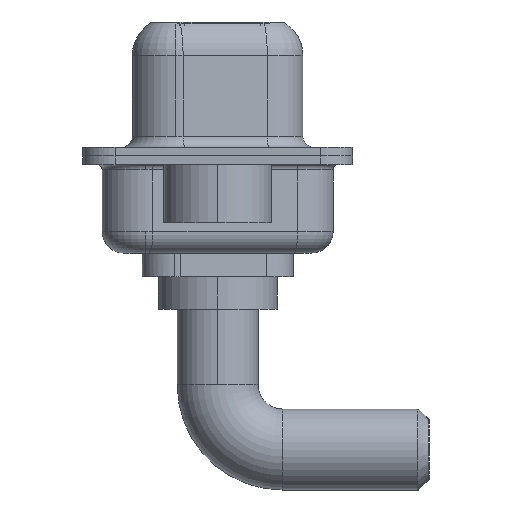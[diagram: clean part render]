
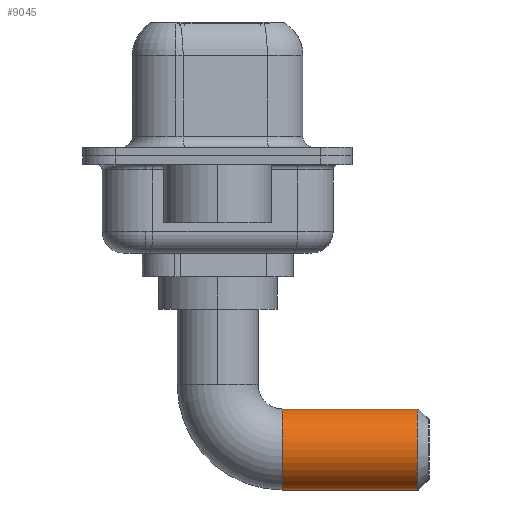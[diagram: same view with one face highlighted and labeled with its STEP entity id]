
A CAD part, left-side view. The second image highlights one B-rep face of the part: STEP entity #9045.
In plain terms, the highlighted cylindrical face has radius 1.875 mm (diameter 3.75 mm), a partial arc.
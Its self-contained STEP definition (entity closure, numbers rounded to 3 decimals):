
#476 = FACE_OUTER_BOUND ( 'NONE', #4622, .T. ) ;
#1003 = DIRECTION ( 'NONE',  ( 0., -1., 0. ) ) ;
#1095 = CARTESIAN_POINT ( 'NONE',  ( 0., -9.25, -6.5 ) ) ;
#1672 = DIRECTION ( 'NONE',  ( 0., -1., 0. ) ) ;
#1710 = AXIS2_PLACEMENT_3D ( 'NONE', #13670, #1672, #4102 ) ;
#2122 = LINE ( 'NONE', #7377, #5929 ) ;
#2336 = DIRECTION ( 'NONE',  ( 0., -1., 0. ) ) ;
#3312 = VERTEX_POINT ( 'NONE', #9047 ) ;
#3387 = LINE ( 'NONE', #7659, #5757 ) ;
#3715 = ORIENTED_EDGE ( 'NONE', *, *, #4478, .T. ) ;
#4007 = VERTEX_POINT ( 'NONE', #10687 ) ;
#4102 = DIRECTION ( 'NONE',  ( 0., 0., -1. ) ) ;
#4448 = DIRECTION ( 'NONE',  ( 0., 1., 0. ) ) ;
#4478 = EDGE_CURVE ( 'NONE', #13500, #13512, #5215, .T. ) ;
#4620 = CIRCLE ( 'NONE', #13325, 1.875 ) ;
#4622 = EDGE_LOOP ( 'NONE', ( #6902, #12253, #5522, #3715 ) ) ;
#5215 = CIRCLE ( 'NONE', #10557, 1.875 ) ;
#5522 = ORIENTED_EDGE ( 'NONE', *, *, #8245, .T. ) ;
#5757 = VECTOR ( 'NONE', #2336, 1000. ) ;
#5866 = CYLINDRICAL_SURFACE ( 'NONE', #1710, 1.875 ) ;
#5929 = VECTOR ( 'NONE', #1003, 1000. ) ;
#6902 = ORIENTED_EDGE ( 'NONE', *, *, #10692, .F. ) ;
#7173 = CARTESIAN_POINT ( 'NONE',  ( 0., -9.25, -4.625 ) ) ;
#7309 = DIRECTION ( 'NONE',  ( -1., 0., 0. ) ) ;
#7377 = CARTESIAN_POINT ( 'NONE',  ( 0., -3., -8.375 ) ) ;
#7444 = DIRECTION ( 'NONE',  ( 0., -1., 0. ) ) ;
#7659 = CARTESIAN_POINT ( 'NONE',  ( 0., -3., -4.625 ) ) ;
#8245 = EDGE_CURVE ( 'NONE', #3312, #13500, #2122, .T. ) ;
#8360 = CARTESIAN_POINT ( 'NONE',  ( 0., -9.25, -8.375 ) ) ;
#8423 = CARTESIAN_POINT ( 'NONE',  ( 0., -3., -6.5 ) ) ;
#9045 = ADVANCED_FACE ( 'NONE', ( #476 ), #5866, .T. ) ;
#9047 = CARTESIAN_POINT ( 'NONE',  ( 0., -3., -8.375 ) ) ;
#10557 = AXIS2_PLACEMENT_3D ( 'NONE', #1095, #4448, #12777 ) ;
#10687 = CARTESIAN_POINT ( 'NONE',  ( 0., -3., -4.625 ) ) ;
#10692 = EDGE_CURVE ( 'NONE', #4007, #13512, #3387, .T. ) ;
#11068 = EDGE_CURVE ( 'NONE', #4007, #3312, #4620, .T. ) ;
#12253 = ORIENTED_EDGE ( 'NONE', *, *, #11068, .T. ) ;
#12777 = DIRECTION ( 'NONE',  ( 0., 0., -1. ) ) ;
#13325 = AXIS2_PLACEMENT_3D ( 'NONE', #8423, #7444, #7309 ) ;
#13500 = VERTEX_POINT ( 'NONE', #8360 ) ;
#13512 = VERTEX_POINT ( 'NONE', #7173 ) ;
#13670 = CARTESIAN_POINT ( 'NONE',  ( 0., -3., -6.5 ) ) ;
